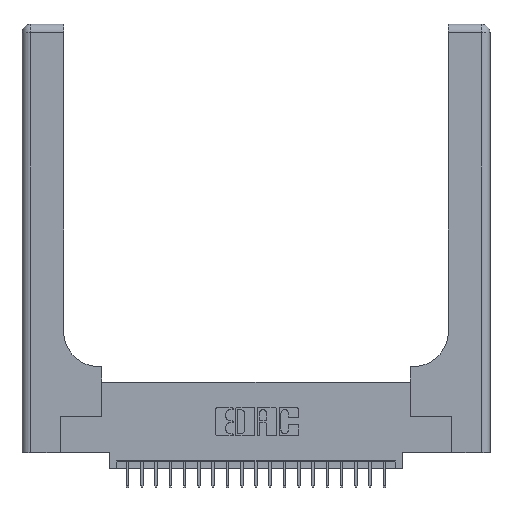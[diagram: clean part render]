
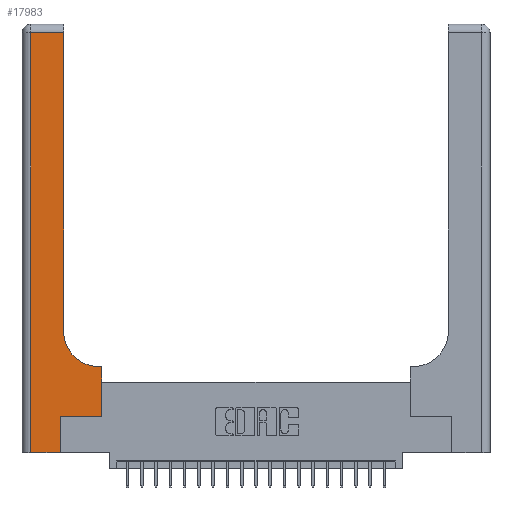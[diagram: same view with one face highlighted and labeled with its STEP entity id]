
A CAD part, top view. The second image highlights one B-rep face of the part: STEP entity #17983.
In plain terms, the highlighted planar face has unit normal (0, 0, 1).
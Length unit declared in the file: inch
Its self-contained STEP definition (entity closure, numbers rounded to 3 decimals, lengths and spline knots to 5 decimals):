
#319 = DIRECTION ( 'NONE',  ( 0., 1., 0. ) ) ;
#426 = ORIENTED_EDGE ( 'NONE', *, *, #14340, .T. ) ;
#517 = VERTEX_POINT ( 'NONE', #17626 ) ;
#1291 = AXIS2_PLACEMENT_3D ( 'NONE', #15509, #19293, #22838 ) ;
#1604 = CARTESIAN_POINT ( 'NONE',  ( 0.5585, 0.25, 0.37 ) ) ;
#1856 = ORIENTED_EDGE ( 'NONE', *, *, #7193, .T. ) ;
#2229 = CARTESIAN_POINT ( 'NONE',  ( 0.269, 0., 0.37 ) ) ;
#2288 = LINE ( 'NONE', #6079, #16183 ) ;
#3460 = LINE ( 'NONE', #8923, #5298 ) ;
#3632 = DIRECTION ( 'NONE',  ( 0., 1., 0. ) ) ;
#4136 = CARTESIAN_POINT ( 'NONE',  ( 0.5415, 0.85, 0.37 ) ) ;
#4464 = VERTEX_POINT ( 'NONE', #17653 ) ;
#4630 = EDGE_CURVE ( 'NONE', #20286, #517, #20239, .T. ) ;
#5096 = ORIENTED_EDGE ( 'NONE', *, *, #14940, .T. ) ;
#5298 = VECTOR ( 'NONE', #19824, 39.37008 ) ;
#5412 = LINE ( 'NONE', #14441, #16683 ) ;
#6008 = CARTESIAN_POINT ( 'NONE',  ( 0., 2.94, 0.37 ) ) ;
#6079 = CARTESIAN_POINT ( 'NONE',  ( 0.269, 0.25, 0.37 ) ) ;
#6127 = LINE ( 'NONE', #6008, #8824 ) ;
#7193 = EDGE_CURVE ( 'NONE', #517, #9691, #5412, .T. ) ;
#7556 = CIRCLE ( 'NONE', #16666, 0.25 ) ;
#7700 = DIRECTION ( 'NONE',  ( 1., 0., 0. ) ) ;
#7890 = VECTOR ( 'NONE', #319, 39.37008 ) ;
#8045 = CARTESIAN_POINT ( 'NONE',  ( 0.5585, 0.25, 0.37 ) ) ;
#8295 = CARTESIAN_POINT ( 'NONE',  ( 0.06, 0., 0.37 ) ) ;
#8467 = ORIENTED_EDGE ( 'NONE', *, *, #9375, .T. ) ;
#8792 = EDGE_CURVE ( 'NONE', #21358, #13128, #19043, .T. ) ;
#8824 = VECTOR ( 'NONE', #18824, 39.37008 ) ;
#8923 = CARTESIAN_POINT ( 'NONE',  ( 0.06, 3., 0.37 ) ) ;
#9189 = LINE ( 'NONE', #22213, #20595 ) ;
#9375 = EDGE_CURVE ( 'NONE', #17497, #15832, #3460, .T. ) ;
#9691 = VERTEX_POINT ( 'NONE', #18511 ) ;
#9738 = ORIENTED_EDGE ( 'NONE', *, *, #22415, .T. ) ;
#10022 = CARTESIAN_POINT ( 'NONE',  ( 0.2915, 3., 0.37 ) ) ;
#10896 = LINE ( 'NONE', #2229, #7890 ) ;
#11043 = CARTESIAN_POINT ( 'NONE',  ( 0.06, 2.94, 0.37 ) ) ;
#11722 = FACE_OUTER_BOUND ( 'NONE', #18503, .T. ) ;
#12085 = PLANE ( 'NONE',  #1291 ) ;
#13128 = VERTEX_POINT ( 'NONE', #17587 ) ;
#13289 = DIRECTION ( 'NONE',  ( 0., 0., -1. ) ) ;
#13781 = ORIENTED_EDGE ( 'NONE', *, *, #16502, .T. ) ;
#14340 = EDGE_CURVE ( 'NONE', #9691, #21358, #7556, .T. ) ;
#14441 = CARTESIAN_POINT ( 'NONE',  ( 0.2915, 0.6, 0.37 ) ) ;
#14940 = EDGE_CURVE ( 'NONE', #13128, #17497, #6127, .T. ) ;
#15089 = DIRECTION ( 'NONE',  ( 1., 0., 0. ) ) ;
#15509 = CARTESIAN_POINT ( 'NONE',  ( 0., 3., 0.37 ) ) ;
#15832 = VERTEX_POINT ( 'NONE', #8295 ) ;
#16183 = VECTOR ( 'NONE', #15089, 39.37008 ) ;
#16207 = VECTOR ( 'NONE', #3632, 39.37008 ) ;
#16502 = EDGE_CURVE ( 'NONE', #15832, #4464, #9189, .T. ) ;
#16666 = AXIS2_PLACEMENT_3D ( 'NONE', #4136, #13289, #7700 ) ;
#16683 = VECTOR ( 'NONE', #21656, 39.37008 ) ;
#17127 = ORIENTED_EDGE ( 'NONE', *, *, #20988, .T. ) ;
#17397 = DIRECTION ( 'NONE',  ( 0., 1., 0. ) ) ;
#17497 = VERTEX_POINT ( 'NONE', #11043 ) ;
#17587 = CARTESIAN_POINT ( 'NONE',  ( 0.2915, 2.94, 0.37 ) ) ;
#17626 = CARTESIAN_POINT ( 'NONE',  ( 0.5585, 0.6, 0.37 ) ) ;
#17653 = CARTESIAN_POINT ( 'NONE',  ( 0.269, 0., 0.37 ) ) ;
#17983 = ADVANCED_FACE ( 'NONE', ( #11722 ), #12085, .F. ) ;
#18281 = CARTESIAN_POINT ( 'NONE',  ( 0.269, 0.25, 0.37 ) ) ;
#18412 = ORIENTED_EDGE ( 'NONE', *, *, #8792, .T. ) ;
#18503 = EDGE_LOOP ( 'NONE', ( #18412, #5096, #8467, #13781, #9738, #17127, #22342, #1856, #426 ) ) ;
#18511 = CARTESIAN_POINT ( 'NONE',  ( 0.5415, 0.6, 0.37 ) ) ;
#18671 = VERTEX_POINT ( 'NONE', #18281 ) ;
#18824 = DIRECTION ( 'NONE',  ( -1., 0., 0. ) ) ;
#19043 = LINE ( 'NONE', #10022, #22685 ) ;
#19293 = DIRECTION ( 'NONE',  ( 0., 0., -1. ) ) ;
#19824 = DIRECTION ( 'NONE',  ( 0., -1., 0. ) ) ;
#19987 = DIRECTION ( 'NONE',  ( 1., 0., 0. ) ) ;
#20239 = LINE ( 'NONE', #1604, #16207 ) ;
#20286 = VERTEX_POINT ( 'NONE', #8045 ) ;
#20595 = VECTOR ( 'NONE', #19987, 39.37008 ) ;
#20988 = EDGE_CURVE ( 'NONE', #18671, #20286, #2288, .T. ) ;
#21358 = VERTEX_POINT ( 'NONE', #22246 ) ;
#21656 = DIRECTION ( 'NONE',  ( -1., 0., 0. ) ) ;
#22213 = CARTESIAN_POINT ( 'NONE',  ( 0., 0., 0.37 ) ) ;
#22246 = CARTESIAN_POINT ( 'NONE',  ( 0.2915, 0.85, 0.37 ) ) ;
#22342 = ORIENTED_EDGE ( 'NONE', *, *, #4630, .T. ) ;
#22415 = EDGE_CURVE ( 'NONE', #4464, #18671, #10896, .T. ) ;
#22685 = VECTOR ( 'NONE', #17397, 39.37008 ) ;
#22838 = DIRECTION ( 'NONE',  ( -1., 0., 0. ) ) ;
